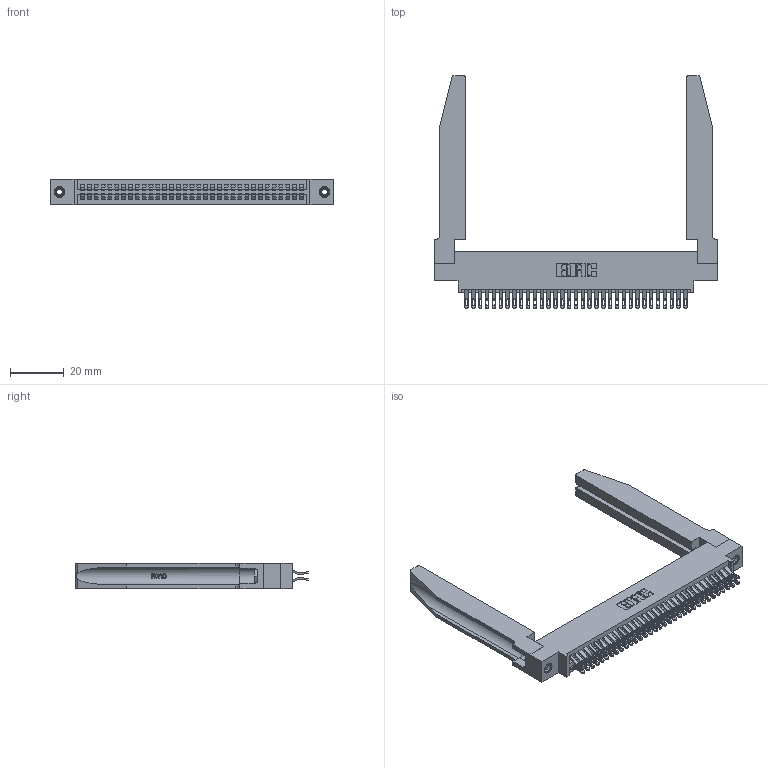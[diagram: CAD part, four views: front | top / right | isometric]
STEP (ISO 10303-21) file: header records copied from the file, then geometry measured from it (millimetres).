
FILE_DESCRIPTION (( 'STEP AP203' ), '1' );
FILE_NAME ('345-066-555-878.STEP', '2019-10-30T18:03:58', ( '' ), ( '' ), 'SwSTEP 2.0', 'SolidWorks 2016', '' );
FILE_SCHEMA (( 'CONFIG_CONTROL_DESIGN' ));
Length unit declared in the file: inch
Products named in the file (5): 345-250-001_345-250-001-102; 345-220-078_345-220-078; 345-066-555-878; 345 Part_0.170 Offset - 0.156 Dia-TH; 345-292-001_555 Tail
Assembly tree (71 placements, depth 2):
  345-066-555-878
    345 Part_0.170 Offset - 0.156 Dia-TH
    345-292-001_555 Tail  x66
    345-250-001_345-250-001-102  x2
    345-220-078_345-220-078  x2
Bounding box: 105.05 x 86.41 x 9.4 mm (x, y, z)
Volume: 17970 mm3; surface area: 22550.2 mm2
Topology: 71 solids, 71 shells, 4060 faces, 12643 edges, 8418 vertices
Faces by surface type: plane 2272, cylinder 1736, bspline 36, cone 12, torus 4
Entity records: 32302 total; most frequent: CARTESIAN_POINT 6377, ORIENTED_EDGE 5178, DIRECTION 4595, EDGE_CURVE 2589, LINE 2211, VECTOR 2211, VERTEX_POINT 1720, AXIS2_PLACEMENT_3D 1192
